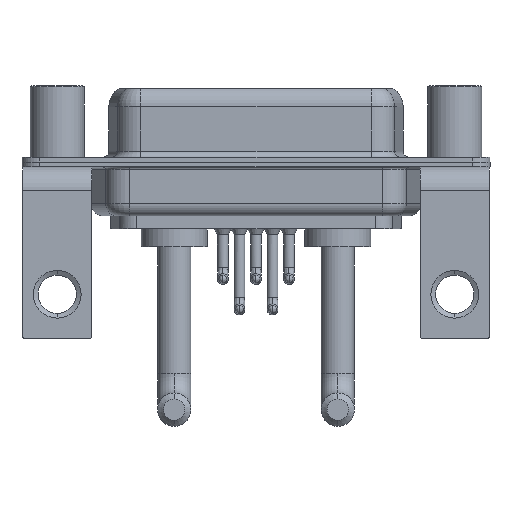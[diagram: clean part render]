
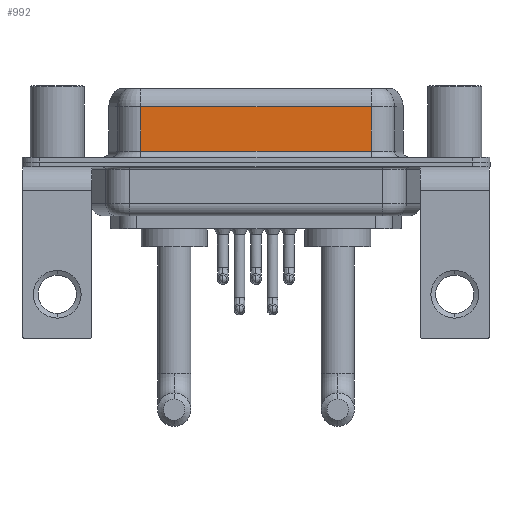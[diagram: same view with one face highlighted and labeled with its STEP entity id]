
A CAD part, front view. The second image highlights one B-rep face of the part: STEP entity #992.
In plain terms, the highlighted planar face has unit normal (0, -1, 0).
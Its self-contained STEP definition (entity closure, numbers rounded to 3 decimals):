
#155 = VECTOR ( 'NONE', #16713, 1000. ) ;
#930 = LINE ( 'NONE', #17047, #14751 ) ;
#992 = ADVANCED_FACE ( 'NONE', ( #16890 ), #1505, .F. ) ;
#1450 = CARTESIAN_POINT ( 'NONE',  ( 26.287, -3.95, 0.9 ) ) ;
#1505 = PLANE ( 'NONE',  #15374 ) ;
#1939 = EDGE_CURVE ( 'NONE', #5022, #12665, #3212, .T. ) ;
#2621 = ORIENTED_EDGE ( 'NONE', *, *, #14629, .F. ) ;
#3212 = LINE ( 'NONE', #6342, #18132 ) ;
#3851 = DIRECTION ( 'NONE',  ( 1., 0., 0. ) ) ;
#4349 = DIRECTION ( 'NONE',  ( 0., 1., 0. ) ) ;
#4498 = VERTEX_POINT ( 'NONE', #8964 ) ;
#5022 = VERTEX_POINT ( 'NONE', #10222 ) ;
#6342 = CARTESIAN_POINT ( 'NONE',  ( 26.287, -3.95, 4.65 ) ) ;
#6916 = DIRECTION ( 'NONE',  ( 0., 0., -1. ) ) ;
#7337 = ORIENTED_EDGE ( 'NONE', *, *, #7875, .T. ) ;
#7875 = EDGE_CURVE ( 'NONE', #4498, #12044, #9760, .T. ) ;
#7917 = DIRECTION ( 'NONE',  ( -1., 0., 0. ) ) ;
#8964 = CARTESIAN_POINT ( 'NONE',  ( 7.013, -3.95, 0.9 ) ) ;
#9652 = ORIENTED_EDGE ( 'NONE', *, *, #10171, .T. ) ;
#9760 = LINE ( 'NONE', #17305, #18839 ) ;
#10171 = EDGE_CURVE ( 'NONE', #12665, #4498, #930, .T. ) ;
#10222 = CARTESIAN_POINT ( 'NONE',  ( 26.287, -3.95, 4.65 ) ) ;
#10738 = CARTESIAN_POINT ( 'NONE',  ( 26.287, -3.95, 6.4 ) ) ;
#12044 = VERTEX_POINT ( 'NONE', #1450 ) ;
#12372 = DIRECTION ( 'NONE',  ( 0., 0., 1. ) ) ;
#12665 = VERTEX_POINT ( 'NONE', #14653 ) ;
#12836 = ORIENTED_EDGE ( 'NONE', *, *, #1939, .T. ) ;
#14629 = EDGE_CURVE ( 'NONE', #5022, #12044, #18193, .T. ) ;
#14653 = CARTESIAN_POINT ( 'NONE',  ( 7.013, -3.95, 4.65 ) ) ;
#14751 = VECTOR ( 'NONE', #6916, 1000. ) ;
#14834 = CARTESIAN_POINT ( 'NONE',  ( 26.287, -3.95, 6.4 ) ) ;
#15374 = AXIS2_PLACEMENT_3D ( 'NONE', #14834, #4349, #12372 ) ;
#16713 = DIRECTION ( 'NONE',  ( 0., 0., -1. ) ) ;
#16890 = FACE_OUTER_BOUND ( 'NONE', #17460, .T. ) ;
#17047 = CARTESIAN_POINT ( 'NONE',  ( 7.013, -3.95, 6.4 ) ) ;
#17305 = CARTESIAN_POINT ( 'NONE',  ( 26.287, -3.95, 0.9 ) ) ;
#17460 = EDGE_LOOP ( 'NONE', ( #2621, #12836, #9652, #7337 ) ) ;
#18132 = VECTOR ( 'NONE', #7917, 1000. ) ;
#18193 = LINE ( 'NONE', #10738, #155 ) ;
#18839 = VECTOR ( 'NONE', #3851, 1000. ) ;
